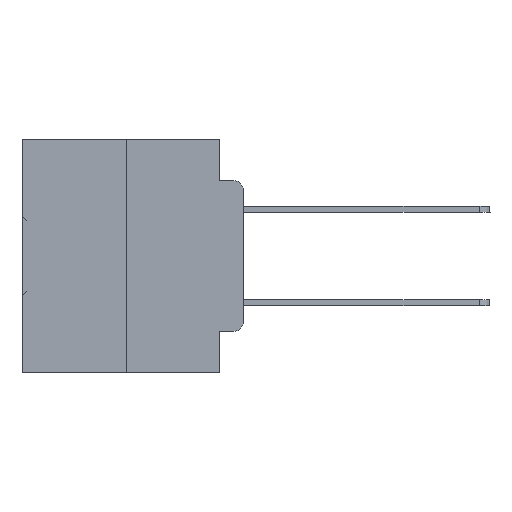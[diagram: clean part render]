
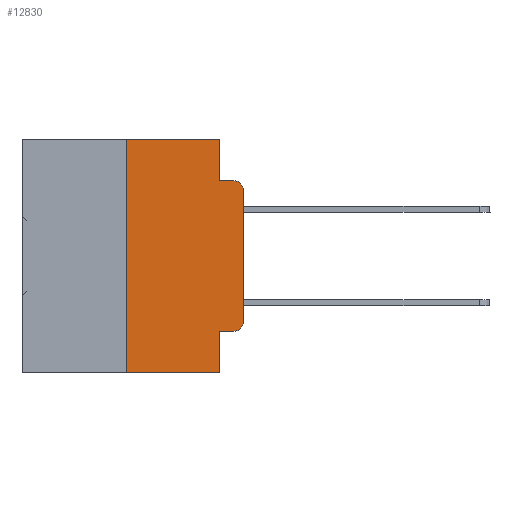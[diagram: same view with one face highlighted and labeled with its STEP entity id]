
A CAD part, left-side view. The second image highlights one B-rep face of the part: STEP entity #12830.
In plain terms, the highlighted planar face has unit normal (-1, 0, 0).
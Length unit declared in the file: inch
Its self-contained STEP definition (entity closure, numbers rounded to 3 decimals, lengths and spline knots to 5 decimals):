
#50 = DIRECTION ( 'NONE',  ( 0., 0., 1. ) ) ;
#368 = LINE ( 'NONE', #14628, #8429 ) ;
#506 = CARTESIAN_POINT ( 'NONE',  ( 0., 0., -0.1085 ) ) ;
#963 = CARTESIAN_POINT ( 'NONE',  ( 0., 0.051, -0.4115 ) ) ;
#1219 = LINE ( 'NONE', #35938, #30275 ) ;
#1691 = DIRECTION ( 'NONE',  ( 0., 0., -1. ) ) ;
#2100 = CARTESIAN_POINT ( 'NONE',  ( 0., 0.051, -0.4115 ) ) ;
#2278 = VERTEX_POINT ( 'NONE', #2100 ) ;
#2558 = ORIENTED_EDGE ( 'NONE', *, *, #13902, .F. ) ;
#2651 = LINE ( 'NONE', #29504, #3530 ) ;
#2685 = DIRECTION ( 'NONE',  ( 0., -1., 0. ) ) ;
#2693 = VERTEX_POINT ( 'NONE', #27162 ) ;
#2851 = ORIENTED_EDGE ( 'NONE', *, *, #32411, .T. ) ;
#2891 = ORIENTED_EDGE ( 'NONE', *, *, #15157, .F. ) ;
#3515 = AXIS2_PLACEMENT_3D ( 'NONE', #9053, #26039, #17811 ) ;
#3530 = VECTOR ( 'NONE', #29878, 39.37008 ) ;
#3860 = VECTOR ( 'NONE', #30464, 39.37008 ) ;
#3875 = VERTEX_POINT ( 'NONE', #8787 ) ;
#4085 = VECTOR ( 'NONE', #14083, 39.37008 ) ;
#4342 = CARTESIAN_POINT ( 'NONE',  ( 0., 0.051, -0.0885 ) ) ;
#4681 = CARTESIAN_POINT ( 'NONE',  ( 0., 0.25, -0.5 ) ) ;
#5382 = CARTESIAN_POINT ( 'NONE',  ( 0., 0.051, 0. ) ) ;
#5646 = CARTESIAN_POINT ( 'NONE',  ( 0., 0.473, 0. ) ) ;
#5841 = LINE ( 'NONE', #31657, #28218 ) ;
#6135 = EDGE_CURVE ( 'NONE', #20514, #2693, #1219, .T. ) ;
#6844 = CARTESIAN_POINT ( 'NONE',  ( 0., 0., -0.3915 ) ) ;
#7866 = AXIS2_PLACEMENT_3D ( 'NONE', #5646, #14295, #34288 ) ;
#8429 = VECTOR ( 'NONE', #17141, 39.37008 ) ;
#8787 = CARTESIAN_POINT ( 'NONE',  ( 0., 0.02, -0.4115 ) ) ;
#9053 = CARTESIAN_POINT ( 'NONE',  ( 0., 0.02, -0.3915 ) ) ;
#9575 = LINE ( 'NONE', #5382, #10494 ) ;
#10494 = VECTOR ( 'NONE', #25142, 39.37008 ) ;
#11315 = CARTESIAN_POINT ( 'NONE',  ( 0., 0.473, 0. ) ) ;
#12830 = ADVANCED_FACE ( 'NONE', ( #35924 ), #22820, .F. ) ;
#13280 = LINE ( 'NONE', #963, #3860 ) ;
#13902 = EDGE_CURVE ( 'NONE', #20449, #22664, #36281, .T. ) ;
#14083 = DIRECTION ( 'NONE',  ( 0., 0., -1. ) ) ;
#14295 = DIRECTION ( 'NONE',  ( 1., 0., 0. ) ) ;
#14628 = CARTESIAN_POINT ( 'NONE',  ( 0., 0.25, 0. ) ) ;
#15157 = EDGE_CURVE ( 'NONE', #2278, #33537, #9575, .T. ) ;
#16564 = ORIENTED_EDGE ( 'NONE', *, *, #36195, .T. ) ;
#17141 = DIRECTION ( 'NONE',  ( 0., 0., 1. ) ) ;
#17524 = LINE ( 'NONE', #23099, #4085 ) ;
#17811 = DIRECTION ( 'NONE',  ( 0., 0., -1. ) ) ;
#18713 = DIRECTION ( 'NONE',  ( -1., 0., 0. ) ) ;
#18736 = ORIENTED_EDGE ( 'NONE', *, *, #32020, .T. ) ;
#19111 = DIRECTION ( 'NONE',  ( 0., -1., 0. ) ) ;
#19188 = ORIENTED_EDGE ( 'NONE', *, *, #31867, .F. ) ;
#19851 = CARTESIAN_POINT ( 'NONE',  ( 0., 0.051, -0.5 ) ) ;
#20449 = VERTEX_POINT ( 'NONE', #24239 ) ;
#20514 = VERTEX_POINT ( 'NONE', #4342 ) ;
#20873 = ORIENTED_EDGE ( 'NONE', *, *, #35352, .F. ) ;
#21081 = ORIENTED_EDGE ( 'NONE', *, *, #28693, .T. ) ;
#21632 = AXIS2_PLACEMENT_3D ( 'NONE', #35783, #18713, #1691 ) ;
#21655 = ORIENTED_EDGE ( 'NONE', *, *, #34885, .T. ) ;
#22049 = CIRCLE ( 'NONE', #3515, 0.02 ) ;
#22664 = VERTEX_POINT ( 'NONE', #36368 ) ;
#22820 = PLANE ( 'NONE',  #7866 ) ;
#23099 = CARTESIAN_POINT ( 'NONE',  ( 0., 0.051, 0. ) ) ;
#24239 = CARTESIAN_POINT ( 'NONE',  ( 0., 0.25, 0. ) ) ;
#24310 = ORIENTED_EDGE ( 'NONE', *, *, #6135, .F. ) ;
#24514 = CIRCLE ( 'NONE', #21632, 0.02 ) ;
#25142 = DIRECTION ( 'NONE',  ( 0., 0., -1. ) ) ;
#25337 = VERTEX_POINT ( 'NONE', #506 ) ;
#26039 = DIRECTION ( 'NONE',  ( -1., 0., 0. ) ) ;
#27162 = CARTESIAN_POINT ( 'NONE',  ( 0., 0.02, -0.0885 ) ) ;
#28218 = VECTOR ( 'NONE', #50, 39.37008 ) ;
#28693 = EDGE_CURVE ( 'NONE', #2278, #3875, #13280, .T. ) ;
#29504 = CARTESIAN_POINT ( 'NONE',  ( 0., 0.473, -0.5 ) ) ;
#29878 = DIRECTION ( 'NONE',  ( 0., -1., 0. ) ) ;
#30275 = VECTOR ( 'NONE', #19111, 39.37008 ) ;
#30464 = DIRECTION ( 'NONE',  ( 0., -1., 0. ) ) ;
#30515 = VECTOR ( 'NONE', #2685, 39.37008 ) ;
#31657 = CARTESIAN_POINT ( 'NONE',  ( 0., 0., 0. ) ) ;
#31867 = EDGE_CURVE ( 'NONE', #22664, #20514, #17524, .T. ) ;
#32020 = EDGE_CURVE ( 'NONE', #3875, #35457, #22049, .T. ) ;
#32411 = EDGE_CURVE ( 'NONE', #35457, #25337, #5841, .T. ) ;
#33537 = VERTEX_POINT ( 'NONE', #19851 ) ;
#34057 = VERTEX_POINT ( 'NONE', #4681 ) ;
#34288 = DIRECTION ( 'NONE',  ( 0., 0., -1. ) ) ;
#34435 = EDGE_LOOP ( 'NONE', ( #2851, #16564, #24310, #19188, #2558, #20873, #21655, #2891, #21081, #18736 ) ) ;
#34885 = EDGE_CURVE ( 'NONE', #34057, #33537, #2651, .T. ) ;
#35352 = EDGE_CURVE ( 'NONE', #34057, #20449, #368, .T. ) ;
#35457 = VERTEX_POINT ( 'NONE', #6844 ) ;
#35783 = CARTESIAN_POINT ( 'NONE',  ( 0., 0.02, -0.1085 ) ) ;
#35924 = FACE_OUTER_BOUND ( 'NONE', #34435, .T. ) ;
#35938 = CARTESIAN_POINT ( 'NONE',  ( 0., 0.051, -0.0885 ) ) ;
#36195 = EDGE_CURVE ( 'NONE', #25337, #2693, #24514, .T. ) ;
#36281 = LINE ( 'NONE', #11315, #30515 ) ;
#36368 = CARTESIAN_POINT ( 'NONE',  ( 0., 0.051, 0. ) ) ;
